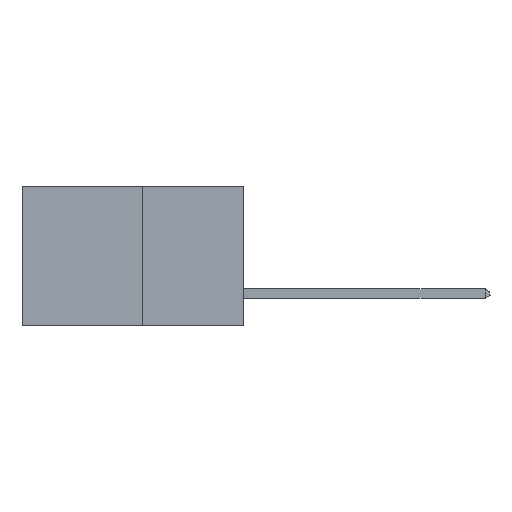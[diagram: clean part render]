
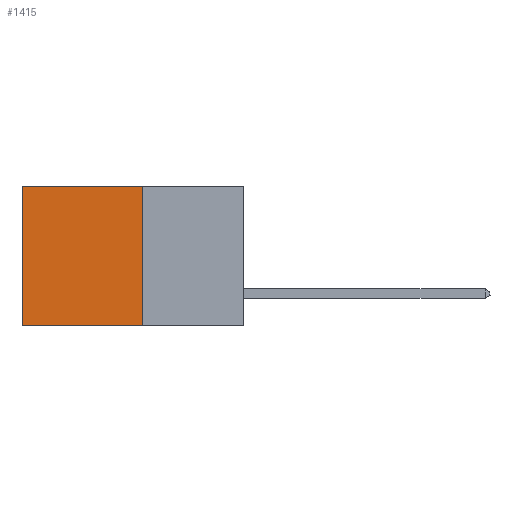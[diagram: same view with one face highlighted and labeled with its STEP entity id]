
A CAD part, left-side view. The second image highlights one B-rep face of the part: STEP entity #1415.
In plain terms, the highlighted planar face has unit normal (-1, 0, 0).
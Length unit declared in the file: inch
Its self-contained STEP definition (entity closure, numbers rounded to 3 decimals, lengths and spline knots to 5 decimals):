
#33 = CARTESIAN_POINT ( 'NONE',  ( 0.277, 0.27, -0.37 ) ) ;
#576 = AXIS2_PLACEMENT_3D ( 'NONE', #1607, #4932, #8353 ) ;
#1245 = VERTEX_POINT ( 'NONE', #12903 ) ;
#1415 = ADVANCED_FACE ( 'NONE', ( #1846 ), #9296, .F. ) ;
#1504 = DIRECTION ( 'NONE',  ( 0., 1., 0. ) ) ;
#1605 = CARTESIAN_POINT ( 'NONE',  ( 0.277, 0.27, -0.37 ) ) ;
#1607 = CARTESIAN_POINT ( 'NONE',  ( 0.277, 0.27, -0.37 ) ) ;
#1846 = FACE_OUTER_BOUND ( 'NONE', #13077, .T. ) ;
#2429 = CARTESIAN_POINT ( 'NONE',  ( 0.277, 0.59, -0.37 ) ) ;
#3167 = CARTESIAN_POINT ( 'NONE',  ( 0.277, 0.59, -0.37 ) ) ;
#3200 = DIRECTION ( 'NONE',  ( 0., 0., -1. ) ) ;
#4223 = ORIENTED_EDGE ( 'NONE', *, *, #8265, .F. ) ;
#4283 = DIRECTION ( 'NONE',  ( 0., 0., -1. ) ) ;
#4794 = VECTOR ( 'NONE', #3200, 39.37008 ) ;
#4932 = DIRECTION ( 'NONE',  ( 1., 0., 0. ) ) ;
#6057 = LINE ( 'NONE', #33, #7890 ) ;
#6088 = CARTESIAN_POINT ( 'NONE',  ( 0.277, 0.27, 0. ) ) ;
#6406 = LINE ( 'NONE', #6088, #8598 ) ;
#7329 = VERTEX_POINT ( 'NONE', #9933 ) ;
#7890 = VECTOR ( 'NONE', #4283, 39.37008 ) ;
#8200 = DIRECTION ( 'NONE',  ( 0., 1., 0. ) ) ;
#8265 = EDGE_CURVE ( 'NONE', #7329, #12500, #13336, .T. ) ;
#8353 = DIRECTION ( 'NONE',  ( 0., 0., -1. ) ) ;
#8598 = VECTOR ( 'NONE', #8200, 39.37008 ) ;
#9296 = PLANE ( 'NONE',  #576 ) ;
#9933 = CARTESIAN_POINT ( 'NONE',  ( 0.277, 0.27, -0.37 ) ) ;
#10082 = EDGE_CURVE ( 'NONE', #13814, #12500, #13626, .T. ) ;
#10464 = ORIENTED_EDGE ( 'NONE', *, *, #10082, .T. ) ;
#10477 = CARTESIAN_POINT ( 'NONE',  ( 0.277, 0.59, 0. ) ) ;
#10588 = VECTOR ( 'NONE', #1504, 39.37008 ) ;
#11204 = ORIENTED_EDGE ( 'NONE', *, *, #12108, .T. ) ;
#11926 = ORIENTED_EDGE ( 'NONE', *, *, #12998, .F. ) ;
#12108 = EDGE_CURVE ( 'NONE', #1245, #13814, #6406, .T. ) ;
#12500 = VERTEX_POINT ( 'NONE', #2429 ) ;
#12903 = CARTESIAN_POINT ( 'NONE',  ( 0.277, 0.27, 0. ) ) ;
#12998 = EDGE_CURVE ( 'NONE', #1245, #7329, #6057, .T. ) ;
#13077 = EDGE_LOOP ( 'NONE', ( #10464, #4223, #11926, #11204 ) ) ;
#13336 = LINE ( 'NONE', #1605, #10588 ) ;
#13626 = LINE ( 'NONE', #3167, #4794 ) ;
#13814 = VERTEX_POINT ( 'NONE', #10477 ) ;
